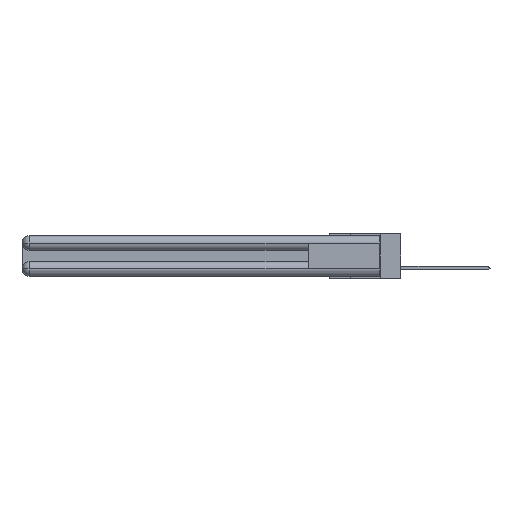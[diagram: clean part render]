
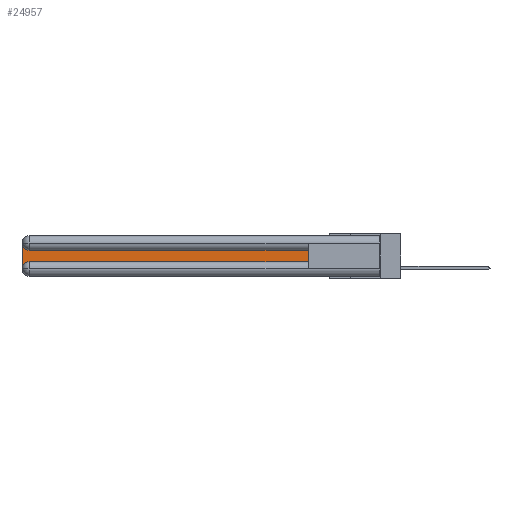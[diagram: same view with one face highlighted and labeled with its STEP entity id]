
A CAD part, left-side view. The second image highlights one B-rep face of the part: STEP entity #24957.
In plain terms, the highlighted planar face has unit normal (-1, 0, 0).
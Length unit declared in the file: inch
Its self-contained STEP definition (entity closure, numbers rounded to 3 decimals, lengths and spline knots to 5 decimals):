
#180 = DIRECTION ( 'NONE',  ( 1., 0., 0. ) ) ;
#566 = LINE ( 'NONE', #21566, #6686 ) ;
#1511 = ORIENTED_EDGE ( 'NONE', *, *, #27240, .T. ) ;
#1563 = CARTESIAN_POINT ( 'NONE',  ( 0.075, 2.94, -0.1225 ) ) ;
#1717 = VERTEX_POINT ( 'NONE', #24866 ) ;
#1994 = CIRCLE ( 'NONE', #10927, 0.06 ) ;
#3033 = ORIENTED_EDGE ( 'NONE', *, *, #12621, .T. ) ;
#3087 = EDGE_CURVE ( 'NONE', #27559, #18921, #1994, .T. ) ;
#4155 = EDGE_CURVE ( 'NONE', #1717, #27655, #18935, .T. ) ;
#4206 = DIRECTION ( 'NONE',  ( 0., 0., 1. ) ) ;
#4769 = AXIS2_PLACEMENT_3D ( 'NONE', #19649, #180, #17740 ) ;
#5794 = VECTOR ( 'NONE', #7441, 39.37008 ) ;
#6316 = ORIENTED_EDGE ( 'NONE', *, *, #8378, .T. ) ;
#6686 = VECTOR ( 'NONE', #8507, 39.37008 ) ;
#6925 = CIRCLE ( 'NONE', #4769, 0.06 ) ;
#7301 = CARTESIAN_POINT ( 'NONE',  ( 0.075, 2.94, -0.2175 ) ) ;
#7441 = DIRECTION ( 'NONE',  ( 0., -1., 0. ) ) ;
#8378 = EDGE_CURVE ( 'NONE', #17456, #27559, #566, .T. ) ;
#8451 = CARTESIAN_POINT ( 'NONE',  ( 0.075, 0.6, -0.2175 ) ) ;
#8507 = DIRECTION ( 'NONE',  ( 0., 0., -1. ) ) ;
#9419 = DIRECTION ( 'NONE',  ( 0., 1., 0. ) ) ;
#9647 = PLANE ( 'NONE',  #19480 ) ;
#10252 = CARTESIAN_POINT ( 'NONE',  ( 0.075, 2.94, -0.2775 ) ) ;
#10508 = EDGE_CURVE ( 'NONE', #27655, #17456, #6925, .T. ) ;
#10927 = AXIS2_PLACEMENT_3D ( 'NONE', #10252, #12718, #12433 ) ;
#11171 = EDGE_LOOP ( 'NONE', ( #27183, #11402, #6316, #19651, #3033, #1511 ) ) ;
#11402 = ORIENTED_EDGE ( 'NONE', *, *, #10508, .T. ) ;
#12183 = VECTOR ( 'NONE', #9419, 39.37008 ) ;
#12433 = DIRECTION ( 'NONE',  ( 0., 0., -1. ) ) ;
#12621 = EDGE_CURVE ( 'NONE', #18921, #15204, #18080, .T. ) ;
#12718 = DIRECTION ( 'NONE',  ( 1., 0., 0. ) ) ;
#14159 = FACE_OUTER_BOUND ( 'NONE', #11171, .T. ) ;
#14206 = DIRECTION ( 'NONE',  ( 1., 0., 0. ) ) ;
#15204 = VERTEX_POINT ( 'NONE', #8451 ) ;
#17456 = VERTEX_POINT ( 'NONE', #20467 ) ;
#17740 = DIRECTION ( 'NONE',  ( 0., 0., -1. ) ) ;
#17880 = VECTOR ( 'NONE', #4206, 39.37008 ) ;
#18080 = LINE ( 'NONE', #18316, #5794 ) ;
#18316 = CARTESIAN_POINT ( 'NONE',  ( 0.075, 0.6, -0.2175 ) ) ;
#18724 = CARTESIAN_POINT ( 'NONE',  ( 0.075, 0.6, -0.1225 ) ) ;
#18921 = VERTEX_POINT ( 'NONE', #7301 ) ;
#18935 = LINE ( 'NONE', #18724, #12183 ) ;
#19480 = AXIS2_PLACEMENT_3D ( 'NONE', #22844, #14206, #24823 ) ;
#19649 = CARTESIAN_POINT ( 'NONE',  ( 0.075, 2.94, -0.0625 ) ) ;
#19651 = ORIENTED_EDGE ( 'NONE', *, *, #3087, .T. ) ;
#20467 = CARTESIAN_POINT ( 'NONE',  ( 0.075, 3., -0.0625 ) ) ;
#21566 = CARTESIAN_POINT ( 'NONE',  ( 0.075, 3., -0.2175 ) ) ;
#22844 = CARTESIAN_POINT ( 'NONE',  ( 0.075, 3., -0.1225 ) ) ;
#23010 = LINE ( 'NONE', #23815, #17880 ) ;
#23655 = CARTESIAN_POINT ( 'NONE',  ( 0.075, 3., -0.2775 ) ) ;
#23815 = CARTESIAN_POINT ( 'NONE',  ( 0.075, 0.6, -0.2175 ) ) ;
#24823 = DIRECTION ( 'NONE',  ( 0., 0., -1. ) ) ;
#24866 = CARTESIAN_POINT ( 'NONE',  ( 0.075, 0.6, -0.1225 ) ) ;
#24957 = ADVANCED_FACE ( 'NONE', ( #14159 ), #9647, .F. ) ;
#27183 = ORIENTED_EDGE ( 'NONE', *, *, #4155, .T. ) ;
#27240 = EDGE_CURVE ( 'NONE', #15204, #1717, #23010, .T. ) ;
#27559 = VERTEX_POINT ( 'NONE', #23655 ) ;
#27655 = VERTEX_POINT ( 'NONE', #1563 ) ;
